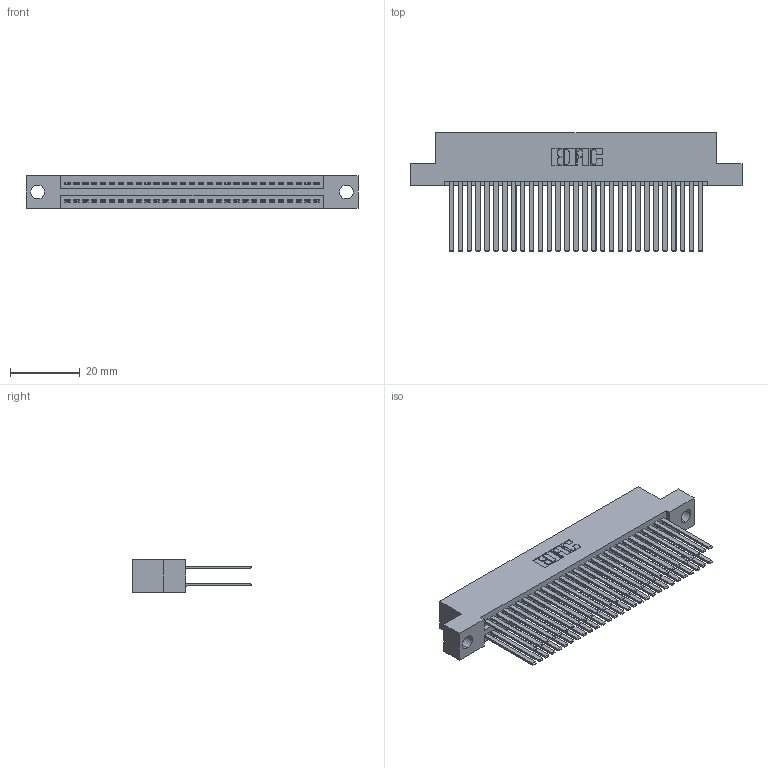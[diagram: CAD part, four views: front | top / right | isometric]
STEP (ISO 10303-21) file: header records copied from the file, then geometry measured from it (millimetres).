
FILE_DESCRIPTION (( 'STEP AP203' ), '1' );
FILE_NAME ('345-058-544-204.STEP', '2018-09-26T15:53:22', ( '' ), ( '' ), 'SwSTEP 2.0', 'SolidWorks 2016', '' );
FILE_SCHEMA (( 'CONFIG_CONTROL_DESIGN' ));
Length unit declared in the file: inch
Products named in the file (3): 345-292-001_345-293-144; 345 Part_Flush Mounting Lugs - 0.156 Dia-TH; 345-058-544-204
Assembly tree (59 placements, depth 2):
  345-058-544-204
    345 Part_Flush Mounting Lugs - 0.156 Dia-TH
    345-292-001_345-293-144  x58
Bounding box: 94.87 x 33.96 x 9.4 mm (x, y, z)
Volume: 9820.2 mm3; surface area: 16462.3 mm2
Topology: 59 solids, 59 shells, 2678 faces, 7939 edges, 5214 vertices
Faces by surface type: plane 1762, cylinder 916
Entity records: 24323 total; most frequent: CARTESIAN_POINT 4088, ORIENTED_EDGE 4022, DIRECTION 3619, EDGE_CURVE 2011, LINE 1767, VECTOR 1767, VERTEX_POINT 1338, AXIS2_PLACEMENT_3D 926
